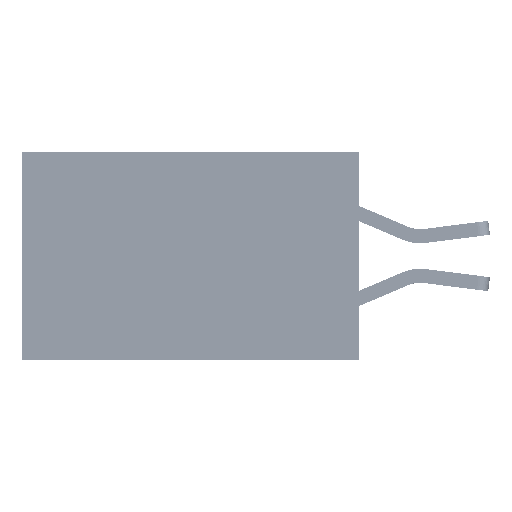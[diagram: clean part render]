
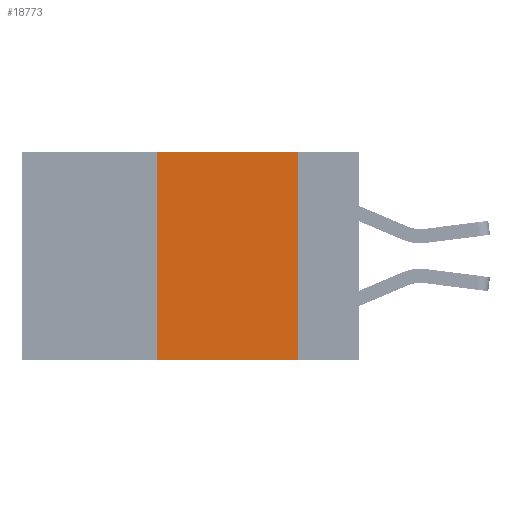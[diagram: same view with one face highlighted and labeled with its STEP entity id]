
A CAD part, left-side view. The second image highlights one B-rep face of the part: STEP entity #18773.
In plain terms, the highlighted planar face has unit normal (-1, 0, 0).
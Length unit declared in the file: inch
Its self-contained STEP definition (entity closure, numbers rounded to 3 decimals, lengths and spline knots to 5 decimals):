
#710 = CARTESIAN_POINT ( 'NONE',  ( 0., 0.6, -0.37 ) ) ;
#734 = CARTESIAN_POINT ( 'NONE',  ( 0., 0.36, 0. ) ) ;
#2647 = FACE_OUTER_BOUND ( 'NONE', #11977, .T. ) ;
#3531 = CARTESIAN_POINT ( 'NONE',  ( 0., 0.11, -0.37 ) ) ;
#6259 = DIRECTION ( 'NONE',  ( 1., 0., 0. ) ) ;
#7173 = AXIS2_PLACEMENT_3D ( 'NONE', #38628, #6259, #38488 ) ;
#9503 = CARTESIAN_POINT ( 'NONE',  ( 0., 0.6, 0. ) ) ;
#10593 = ORIENTED_EDGE ( 'NONE', *, *, #35105, .F. ) ;
#11977 = EDGE_LOOP ( 'NONE', ( #10593, #35454, #25767, #23140 ) ) ;
#12371 = PLANE ( 'NONE',  #7173 ) ;
#12397 = VERTEX_POINT ( 'NONE', #26503 ) ;
#16502 = LINE ( 'NONE', #20760, #23061 ) ;
#18773 = ADVANCED_FACE ( 'NONE', ( #2647 ), #12371, .F. ) ;
#18820 = LINE ( 'NONE', #710, #31470 ) ;
#20760 = CARTESIAN_POINT ( 'NONE',  ( 0., 0.11, 0. ) ) ;
#21420 = EDGE_CURVE ( 'NONE', #40039, #12397, #30287, .T. ) ;
#22067 = VERTEX_POINT ( 'NONE', #27945 ) ;
#22273 = CARTESIAN_POINT ( 'NONE',  ( 0., 0.36, 0. ) ) ;
#23061 = VECTOR ( 'NONE', #36717, 39.37008 ) ;
#23140 = ORIENTED_EDGE ( 'NONE', *, *, #26018, .T. ) ;
#23537 = DIRECTION ( 'NONE',  ( 0., -1., 0. ) ) ;
#25767 = ORIENTED_EDGE ( 'NONE', *, *, #33175, .F. ) ;
#26018 = EDGE_CURVE ( 'NONE', #22067, #28157, #18820, .T. ) ;
#26503 = CARTESIAN_POINT ( 'NONE',  ( 0., 0.11, 0. ) ) ;
#26718 = VECTOR ( 'NONE', #39623, 39.37008 ) ;
#27945 = CARTESIAN_POINT ( 'NONE',  ( 0., 0.36, -0.37 ) ) ;
#28157 = VERTEX_POINT ( 'NONE', #3531 ) ;
#30287 = LINE ( 'NONE', #9503, #36317 ) ;
#31470 = VECTOR ( 'NONE', #23537, 39.37008 ) ;
#33175 = EDGE_CURVE ( 'NONE', #22067, #40039, #35338, .T. ) ;
#35105 = EDGE_CURVE ( 'NONE', #12397, #28157, #16502, .T. ) ;
#35338 = LINE ( 'NONE', #734, #26718 ) ;
#35454 = ORIENTED_EDGE ( 'NONE', *, *, #21420, .F. ) ;
#36317 = VECTOR ( 'NONE', #38326, 39.37008 ) ;
#36717 = DIRECTION ( 'NONE',  ( 0., 0., -1. ) ) ;
#38326 = DIRECTION ( 'NONE',  ( 0., -1., 0. ) ) ;
#38488 = DIRECTION ( 'NONE',  ( 0., 0., -1. ) ) ;
#38628 = CARTESIAN_POINT ( 'NONE',  ( 0., 0.6, 0. ) ) ;
#39623 = DIRECTION ( 'NONE',  ( 0., 0., 1. ) ) ;
#40039 = VERTEX_POINT ( 'NONE', #22273 ) ;
